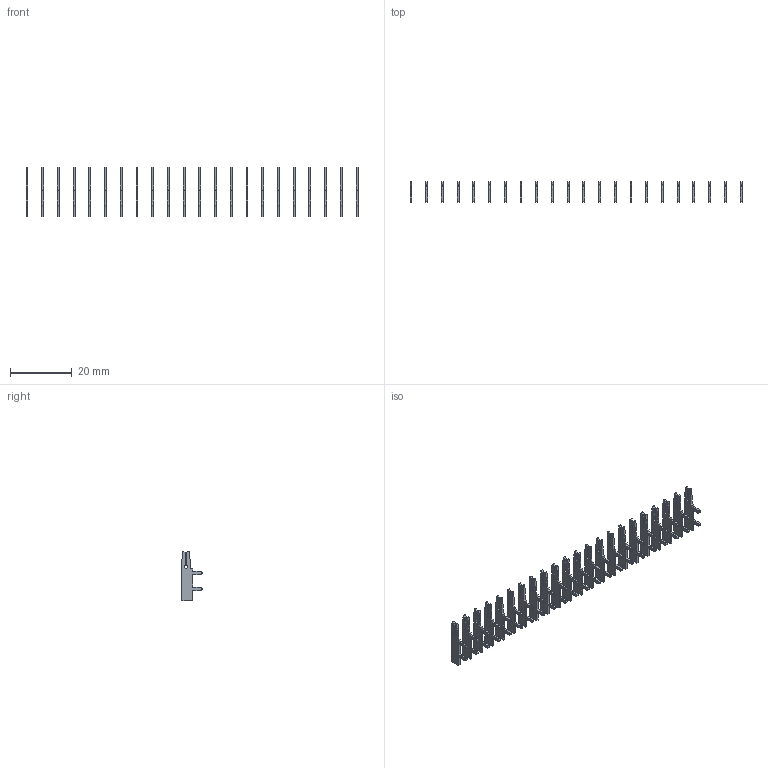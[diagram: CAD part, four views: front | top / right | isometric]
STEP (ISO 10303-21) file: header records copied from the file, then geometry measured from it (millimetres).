
FILE_DESCRIPTION (( 'STEP AP203' ), '1' );
FILE_NAME ('105-022-202-200.STEP', '2020-04-07T23:02:18', ( '' ), ( '' ), 'SwSTEP 2.0', 'SolidWorks 2016', '' );
FILE_SCHEMA (( 'CONFIG_CONTROL_DESIGN' ));
Length unit declared in the file: inch
Products named in the file (2): 100-290-001_100-290-202; 105-022-202-200
Assembly tree (22 placements, depth 2):
  105-022-202-200
    100-290-001_100-290-202  x22
Bounding box: 107.28 x 6.53 x 15.88 mm (x, y, z)
Volume: 699 mm3; surface area: 3108.6 mm2
Topology: 22 solids, 22 shells, 660 faces, 1848 edges, 1232 vertices
Faces by surface type: plane 506, cylinder 154
Entity records: 1834 total; most frequent: CARTESIAN_POINT 207, DIRECTION 204, ORIENTED_EDGE 168, EDGE_CURVE 84, AXIS2_PLACEMENT_3D 69, VECTOR 66, LINE 66, VERTEX_POINT 56
